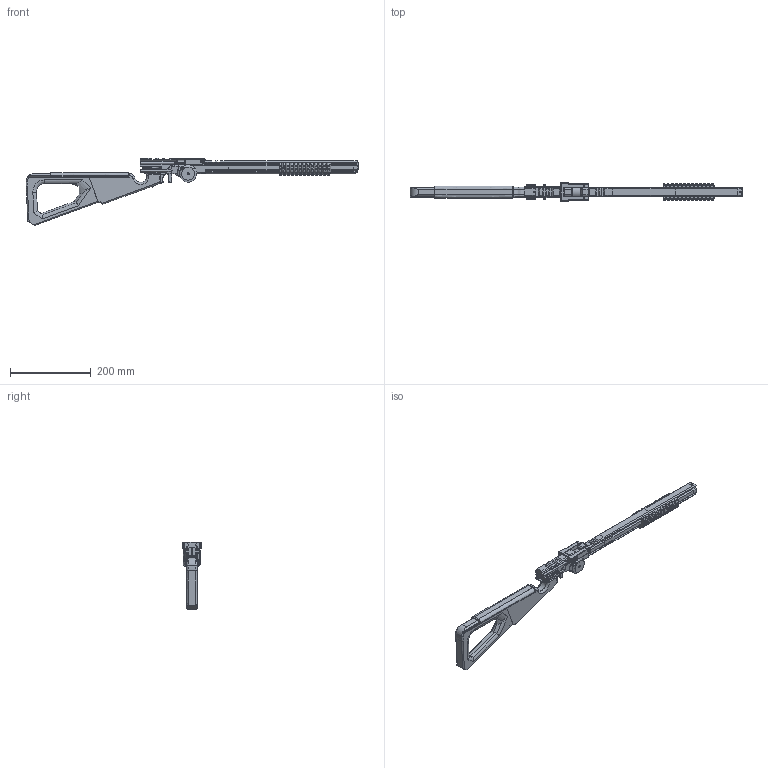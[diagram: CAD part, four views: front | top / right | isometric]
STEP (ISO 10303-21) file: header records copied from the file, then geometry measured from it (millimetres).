
FILE_DESCRIPTION(/* description */ (''),/* implementation_level */ '2;1');
FILE_NAME(/* name */ 'G22_Grizzly_XL.stp',/* time_stamp */ '2020-12-21T10:19:43-06:00',/* author */ (''),/* organization */ (''),/* preprocessor_version */ 'ST-DEVELOPER v15.2',/* originating_system */ 'Autodesk Translator Framework v2.0.0.5431',/* authorisation */ '');
FILE_SCHEMA (('AUTOMOTIVE_DESIGN { 1 0 10303 214 3 1 1 }'));
Products named in the file (1): GrizzlyFinal
Bounding box: 820.96 x 45 x 165.78 mm (x, y, z)
Volume: 880938.2 mm3; surface area: 267745 mm2
Topology: 35 solids, 35 shells, 1806 faces, 4292 edges, 2571 vertices
Faces by surface type: plane 580, cylinder 548, bspline 287, torus 205, sphere 116, cone 70
Full cylindrical faces by diameter (mm): 2.5 x24, 2.855 x1, 2.9 x1, 3 x2, 3.2 x22, 3.7 x1, 3.85 x4, 4.1 x1, 4.25 x8, 4.6 x2, 5 x9, 5.1 x1, 5.5 x1, 6.2 x10, 6.5 x1, 8.3 x4, 8.5 x3, 9.4 x1, 9.5 x1, 10 x1
Entity records: 64236 total; most frequent: CARTESIAN_POINT 24786, DIRECTION 8102, ORIENTED_EDGE 8044, EDGE_CURVE 4022, AXIS2_PLACEMENT_3D 3180, VERTEX_POINT 2528, EDGE_LOOP 2088, ADVANCED_FACE 1799
